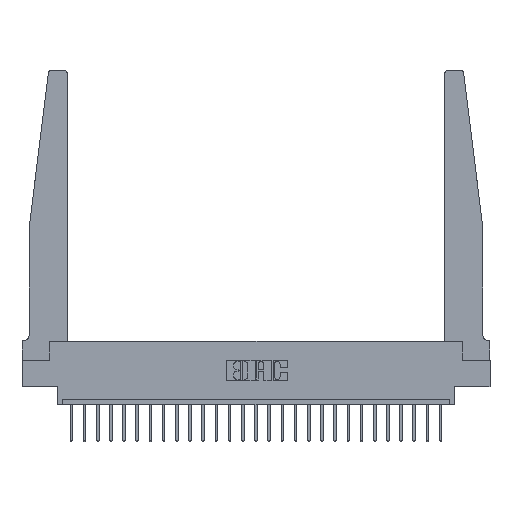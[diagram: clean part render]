
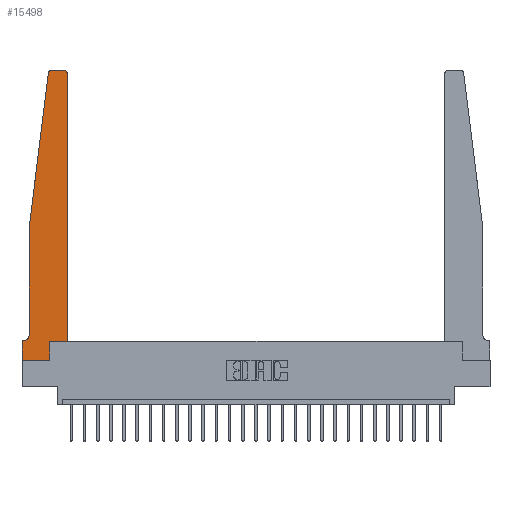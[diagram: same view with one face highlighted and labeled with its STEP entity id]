
A CAD part, top view. The second image highlights one B-rep face of the part: STEP entity #15498.
In plain terms, the highlighted planar face has unit normal (0, 0, 1).
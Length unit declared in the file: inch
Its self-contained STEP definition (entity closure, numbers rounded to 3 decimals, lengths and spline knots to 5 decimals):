
#971 = EDGE_CURVE ( 'NONE', #4050, #15550, #7154, .T. ) ;
#1342 = VECTOR ( 'NONE', #8493, 39.37008 ) ;
#1571 = CIRCLE ( 'NONE', #15163, 0.03 ) ;
#1899 = PLANE ( 'NONE',  #15905 ) ;
#1927 = VERTEX_POINT ( 'NONE', #7102 ) ;
#1956 = ORIENTED_EDGE ( 'NONE', *, *, #19718, .T. ) ;
#2718 = DIRECTION ( 'NONE',  ( 0., -1., 0. ) ) ;
#2987 = EDGE_CURVE ( 'NONE', #9619, #13778, #23747, .T. ) ;
#3012 = CARTESIAN_POINT ( 'NONE',  ( 0., 0., 0.37 ) ) ;
#3147 = CARTESIAN_POINT ( 'NONE',  ( 0.27653, 2.75, 0.37 ) ) ;
#3195 = ORIENTED_EDGE ( 'NONE', *, *, #6256, .T. ) ;
#3363 = DIRECTION ( 'NONE',  ( -0.122, -0.992, 0. ) ) ;
#3435 = CARTESIAN_POINT ( 'NONE',  ( 0.24675, 2.72367, 0.37 ) ) ;
#3463 = DIRECTION ( 'NONE',  ( 0., -1., 0. ) ) ;
#3713 = CARTESIAN_POINT ( 'NONE',  ( 0.015, 0.1875, 0.37 ) ) ;
#3863 = CARTESIAN_POINT ( 'NONE',  ( 0.065, 0.2375, 0.37 ) ) ;
#4050 = VERTEX_POINT ( 'NONE', #3012 ) ;
#4081 = CARTESIAN_POINT ( 'NONE',  ( 0.27653, 2.72, 0.37 ) ) ;
#4176 = CARTESIAN_POINT ( 'NONE',  ( 0.425, 0.18, 0.37 ) ) ;
#4256 = DIRECTION ( 'NONE',  ( 1., 0., 0. ) ) ;
#4310 = DIRECTION ( 'NONE',  ( 1., 0., 0. ) ) ;
#4380 = CARTESIAN_POINT ( 'NONE',  ( 0.425, 2.72, 0.37 ) ) ;
#4711 = VECTOR ( 'NONE', #7107, 39.37008 ) ;
#5420 = LINE ( 'NONE', #22316, #10474 ) ;
#6015 = DIRECTION ( 'NONE',  ( 0., 0., 1. ) ) ;
#6256 = EDGE_CURVE ( 'NONE', #1927, #23409, #9592, .T. ) ;
#6410 = LINE ( 'NONE', #7443, #16501 ) ;
#6500 = EDGE_CURVE ( 'NONE', #21812, #9619, #5420, .T. ) ;
#6686 = CARTESIAN_POINT ( 'NONE',  ( 0.2605, 0.18, 0.37 ) ) ;
#6890 = FACE_OUTER_BOUND ( 'NONE', #18132, .T. ) ;
#7023 = CARTESIAN_POINT ( 'NONE',  ( 0.425, 0.18, 0.37 ) ) ;
#7102 = CARTESIAN_POINT ( 'NONE',  ( 0.425, 0.18, 0.37 ) ) ;
#7107 = DIRECTION ( 'NONE',  ( 1., 0., 0. ) ) ;
#7154 = LINE ( 'NONE', #9838, #16651 ) ;
#7443 = CARTESIAN_POINT ( 'NONE',  ( 0.065, 0.1875, 0.37 ) ) ;
#7459 = ORIENTED_EDGE ( 'NONE', *, *, #971, .T. ) ;
#7634 = LINE ( 'NONE', #6686, #1342 ) ;
#7650 = ORIENTED_EDGE ( 'NONE', *, *, #16259, .T. ) ;
#8080 = ORIENTED_EDGE ( 'NONE', *, *, #2987, .T. ) ;
#8138 = ORIENTED_EDGE ( 'NONE', *, *, #13390, .T. ) ;
#8493 = DIRECTION ( 'NONE',  ( 0., 1., 0. ) ) ;
#8738 = ORIENTED_EDGE ( 'NONE', *, *, #15022, .T. ) ;
#8907 = CARTESIAN_POINT ( 'NONE',  ( 0.065, 1.25, 0.37 ) ) ;
#8988 = VERTEX_POINT ( 'NONE', #12951 ) ;
#9329 = ORIENTED_EDGE ( 'NONE', *, *, #16465, .T. ) ;
#9450 = DIRECTION ( 'NONE',  ( 0., 0., -1. ) ) ;
#9592 = LINE ( 'NONE', #4176, #17307 ) ;
#9619 = VERTEX_POINT ( 'NONE', #3863 ) ;
#9641 = ORIENTED_EDGE ( 'NONE', *, *, #6500, .T. ) ;
#9692 = DIRECTION ( 'NONE',  ( -1., 0., 0. ) ) ;
#9838 = CARTESIAN_POINT ( 'NONE',  ( 0., 0., 0.37 ) ) ;
#9869 = DIRECTION ( 'NONE',  ( 0., 0., 1. ) ) ;
#10083 = LINE ( 'NONE', #21385, #16305 ) ;
#10474 = VECTOR ( 'NONE', #3463, 39.37008 ) ;
#10498 = CARTESIAN_POINT ( 'NONE',  ( 0., 0., 0.37 ) ) ;
#10980 = CARTESIAN_POINT ( 'NONE',  ( 0.065, 1.25, 0.37 ) ) ;
#11164 = AXIS2_PLACEMENT_3D ( 'NONE', #4081, #6015, #13686 ) ;
#12888 = LINE ( 'NONE', #10980, #15515 ) ;
#12951 = CARTESIAN_POINT ( 'NONE',  ( 0.395, 2.75, 0.37 ) ) ;
#12972 = CARTESIAN_POINT ( 'NONE',  ( 0., 0.1875, 0.37 ) ) ;
#13278 = DIRECTION ( 'NONE',  ( 0., 0., 1. ) ) ;
#13390 = EDGE_CURVE ( 'NONE', #8988, #14509, #10083, .T. ) ;
#13686 = DIRECTION ( 'NONE',  ( 1., 0., 0. ) ) ;
#13778 = VERTEX_POINT ( 'NONE', #3713 ) ;
#14509 = VERTEX_POINT ( 'NONE', #3147 ) ;
#15022 = EDGE_CURVE ( 'NONE', #24038, #21812, #12888, .T. ) ;
#15163 = AXIS2_PLACEMENT_3D ( 'NONE', #17432, #9869, #4256 ) ;
#15404 = LINE ( 'NONE', #10498, #16000 ) ;
#15498 = ADVANCED_FACE ( 'NONE', ( #6890 ), #1899, .T. ) ;
#15515 = VECTOR ( 'NONE', #3363, 39.37008 ) ;
#15550 = VERTEX_POINT ( 'NONE', #17827 ) ;
#15705 = DIRECTION ( 'NONE',  ( -1., 0., 0. ) ) ;
#15905 = AXIS2_PLACEMENT_3D ( 'NONE', #16928, #13278, #24562 ) ;
#16000 = VECTOR ( 'NONE', #2718, 39.37008 ) ;
#16259 = EDGE_CURVE ( 'NONE', #14509, #24038, #24097, .T. ) ;
#16305 = VECTOR ( 'NONE', #15705, 39.37008 ) ;
#16465 = EDGE_CURVE ( 'NONE', #24640, #1927, #22313, .T. ) ;
#16501 = VECTOR ( 'NONE', #17659, 39.37008 ) ;
#16651 = VECTOR ( 'NONE', #4310, 39.37008 ) ;
#16928 = CARTESIAN_POINT ( 'NONE',  ( 0., 0.1875, 0.37 ) ) ;
#17004 = AXIS2_PLACEMENT_3D ( 'NONE', #20849, #9450, #9692 ) ;
#17236 = EDGE_CURVE ( 'NONE', #22398, #4050, #15404, .T. ) ;
#17307 = VECTOR ( 'NONE', #19271, 39.37008 ) ;
#17432 = CARTESIAN_POINT ( 'NONE',  ( 0.395, 2.72, 0.37 ) ) ;
#17659 = DIRECTION ( 'NONE',  ( -1., 0., 0. ) ) ;
#17827 = CARTESIAN_POINT ( 'NONE',  ( 0.2605, 0., 0.37 ) ) ;
#18132 = EDGE_LOOP ( 'NONE', ( #8138, #7650, #8738, #9641, #8080, #24429, #22472, #7459, #22502, #9329, #3195, #1956 ) ) ;
#18469 = EDGE_CURVE ( 'NONE', #15550, #24640, #7634, .T. ) ;
#19271 = DIRECTION ( 'NONE',  ( 0., 1., 0. ) ) ;
#19718 = EDGE_CURVE ( 'NONE', #23409, #8988, #1571, .T. ) ;
#19952 = CARTESIAN_POINT ( 'NONE',  ( 0.2605, 0.18, 0.37 ) ) ;
#20849 = CARTESIAN_POINT ( 'NONE',  ( 0.015, 0.2375, 0.37 ) ) ;
#20999 = EDGE_CURVE ( 'NONE', #13778, #22398, #6410, .T. ) ;
#21385 = CARTESIAN_POINT ( 'NONE',  ( 0.25, 2.75, 0.37 ) ) ;
#21812 = VERTEX_POINT ( 'NONE', #8907 ) ;
#22313 = LINE ( 'NONE', #7023, #4711 ) ;
#22316 = CARTESIAN_POINT ( 'NONE',  ( 0.065, 1.25, 0.37 ) ) ;
#22398 = VERTEX_POINT ( 'NONE', #12972 ) ;
#22472 = ORIENTED_EDGE ( 'NONE', *, *, #17236, .T. ) ;
#22502 = ORIENTED_EDGE ( 'NONE', *, *, #18469, .T. ) ;
#23409 = VERTEX_POINT ( 'NONE', #4380 ) ;
#23747 = CIRCLE ( 'NONE', #17004, 0.05 ) ;
#24038 = VERTEX_POINT ( 'NONE', #3435 ) ;
#24097 = CIRCLE ( 'NONE', #11164, 0.03 ) ;
#24429 = ORIENTED_EDGE ( 'NONE', *, *, #20999, .T. ) ;
#24562 = DIRECTION ( 'NONE',  ( 1., 0., 0. ) ) ;
#24640 = VERTEX_POINT ( 'NONE', #19952 ) ;
